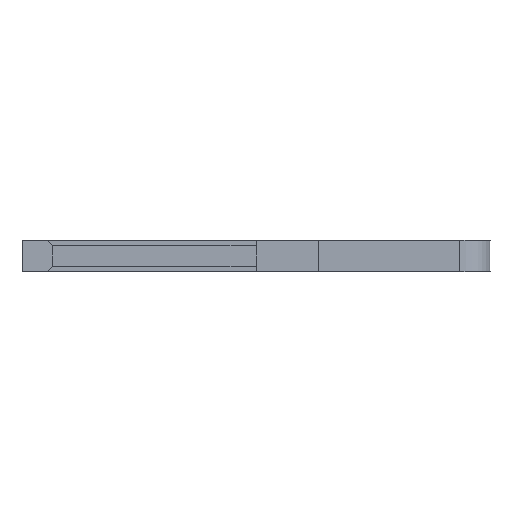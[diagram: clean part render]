
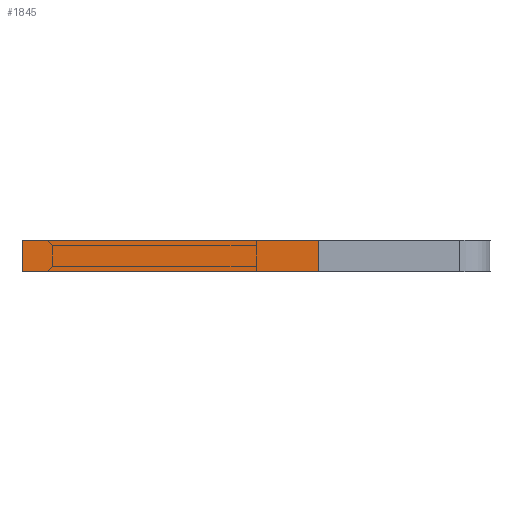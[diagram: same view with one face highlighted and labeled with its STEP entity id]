
A CAD part, left-side view. The second image highlights one B-rep face of the part: STEP entity #1845.
In plain terms, the highlighted face is planar.
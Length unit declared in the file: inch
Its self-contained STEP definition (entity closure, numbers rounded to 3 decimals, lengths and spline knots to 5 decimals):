
#53 = LINE ( 'NONE', #3469, #3342 ) ;
#170 = EDGE_CURVE ( 'NONE', #1675, #665, #2475, .T. ) ;
#182 = DIRECTION ( 'NONE',  ( 0., 1., 0. ) ) ;
#377 = ORIENTED_EDGE ( 'NONE', *, *, #170, .T. ) ;
#405 = VERTEX_POINT ( 'NONE', #4096 ) ;
#428 = DIRECTION ( 'NONE',  ( -1., 0., 0. ) ) ;
#562 = CARTESIAN_POINT ( 'NONE',  ( 0.01, -0.04, -0.04 ) ) ;
#611 = CARTESIAN_POINT ( 'NONE',  ( -0.01, -0.04, -0.04 ) ) ;
#665 = VERTEX_POINT ( 'NONE', #2830 ) ;
#992 = FACE_OUTER_BOUND ( 'NONE', #2717, .T. ) ;
#1071 = DIRECTION ( 'NONE',  ( 0., 1., 0. ) ) ;
#1106 = AXIS2_PLACEMENT_3D ( 'NONE', #1535, #3227, #3848 ) ;
#1128 = VECTOR ( 'NONE', #428, 39.37008 ) ;
#1224 = EDGE_CURVE ( 'NONE', #405, #1947, #53, .T. ) ;
#1535 = CARTESIAN_POINT ( 'NONE',  ( 0.01, 0.15, -0.04 ) ) ;
#1578 = EDGE_CURVE ( 'NONE', #405, #1675, #3017, .T. ) ;
#1585 = VECTOR ( 'NONE', #1071, 39.37008 ) ;
#1675 = VERTEX_POINT ( 'NONE', #611 ) ;
#1680 = CARTESIAN_POINT ( 'NONE',  ( 0.01, 0.15, -0.04 ) ) ;
#1845 = ADVANCED_FACE ( 'NONE', ( #992 ), #2879, .F. ) ;
#1908 = DIRECTION ( 'NONE',  ( -1., 0., 0. ) ) ;
#1947 = VERTEX_POINT ( 'NONE', #3209 ) ;
#2129 = ORIENTED_EDGE ( 'NONE', *, *, #1224, .F. ) ;
#2475 = LINE ( 'NONE', #4065, #1585 ) ;
#2717 = EDGE_LOOP ( 'NONE', ( #377, #3699, #2129, #4001 ) ) ;
#2830 = CARTESIAN_POINT ( 'NONE',  ( -0.01, 0.15, -0.04 ) ) ;
#2879 = PLANE ( 'NONE',  #1106 ) ;
#3017 = LINE ( 'NONE', #562, #3948 ) ;
#3024 = EDGE_CURVE ( 'NONE', #1947, #665, #4066, .T. ) ;
#3209 = CARTESIAN_POINT ( 'NONE',  ( 0.01, 0.15, -0.04 ) ) ;
#3227 = DIRECTION ( 'NONE',  ( 0., 0., 1. ) ) ;
#3342 = VECTOR ( 'NONE', #182, 39.37008 ) ;
#3469 = CARTESIAN_POINT ( 'NONE',  ( 0.01, 0.15, -0.04 ) ) ;
#3699 = ORIENTED_EDGE ( 'NONE', *, *, #3024, .F. ) ;
#3848 = DIRECTION ( 'NONE',  ( 1., 0., 0. ) ) ;
#3948 = VECTOR ( 'NONE', #1908, 39.37008 ) ;
#4001 = ORIENTED_EDGE ( 'NONE', *, *, #1578, .T. ) ;
#4065 = CARTESIAN_POINT ( 'NONE',  ( -0.01, 0.15, -0.04 ) ) ;
#4066 = LINE ( 'NONE', #1680, #1128 ) ;
#4096 = CARTESIAN_POINT ( 'NONE',  ( 0.01, -0.04, -0.04 ) ) ;
